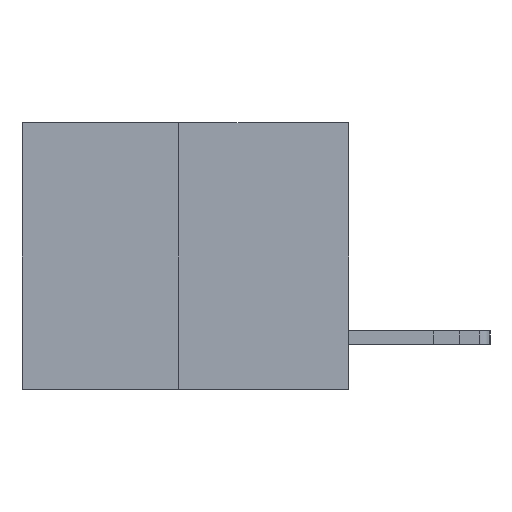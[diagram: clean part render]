
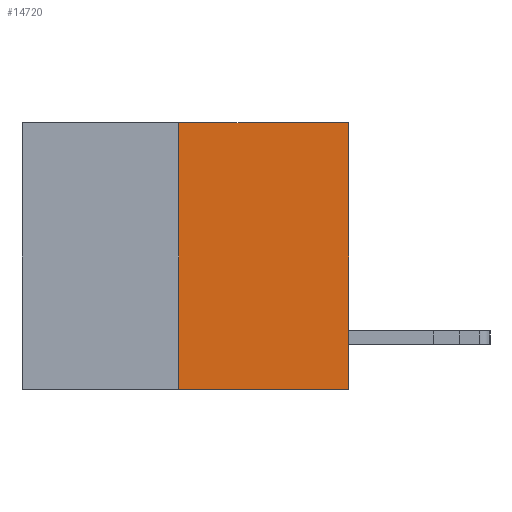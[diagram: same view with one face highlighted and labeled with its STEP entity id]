
A CAD part, left-side view. The second image highlights one B-rep face of the part: STEP entity #14720.
In plain terms, the highlighted planar face has unit normal (-1, 0, 0).
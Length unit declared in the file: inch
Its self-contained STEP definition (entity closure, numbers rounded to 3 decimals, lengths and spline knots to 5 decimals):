
#1725 = EDGE_CURVE ( 'NONE', #3809, #10018, #12631, .T. ) ;
#1791 = CARTESIAN_POINT ( 'NONE',  ( 0., 0.312, 0. ) ) ;
#3809 = VERTEX_POINT ( 'NONE', #7049 ) ;
#4266 = CARTESIAN_POINT ( 'NONE',  ( 0., 0.6, 0. ) ) ;
#4326 = DIRECTION ( 'NONE',  ( 1., 0., 0. ) ) ;
#4959 = ORIENTED_EDGE ( 'NONE', *, *, #5441, .F. ) ;
#5100 = ORIENTED_EDGE ( 'NONE', *, *, #14670, .T. ) ;
#5299 = CARTESIAN_POINT ( 'NONE',  ( 0., 0.6, -0.49 ) ) ;
#5441 = EDGE_CURVE ( 'NONE', #10018, #7235, #14806, .T. ) ;
#5541 = ORIENTED_EDGE ( 'NONE', *, *, #15713, .T. ) ;
#5608 = CARTESIAN_POINT ( 'NONE',  ( 0., 0., -0.49 ) ) ;
#7049 = CARTESIAN_POINT ( 'NONE',  ( 0., 0.312, -0.49 ) ) ;
#7235 = VERTEX_POINT ( 'NONE', #12132 ) ;
#7618 = DIRECTION ( 'NONE',  ( 0., 0., 1. ) ) ;
#7850 = LINE ( 'NONE', #14991, #15889 ) ;
#8002 = CARTESIAN_POINT ( 'NONE',  ( 0., 0.6, 0. ) ) ;
#8866 = VERTEX_POINT ( 'NONE', #5608 ) ;
#9265 = DIRECTION ( 'NONE',  ( 0., 0., -1. ) ) ;
#9460 = LINE ( 'NONE', #5299, #15340 ) ;
#9776 = EDGE_LOOP ( 'NONE', ( #15896, #5100, #5541, #4959 ) ) ;
#10018 = VERTEX_POINT ( 'NONE', #1791 ) ;
#10072 = DIRECTION ( 'NONE',  ( 0., 0., 1. ) ) ;
#10525 = CARTESIAN_POINT ( 'NONE',  ( 0., 0.312, -0.49 ) ) ;
#10681 = VECTOR ( 'NONE', #15390, 39.37008 ) ;
#11904 = PLANE ( 'NONE',  #14398 ) ;
#12132 = CARTESIAN_POINT ( 'NONE',  ( 0., 0., 0. ) ) ;
#12631 = LINE ( 'NONE', #10525, #13017 ) ;
#12973 = FACE_OUTER_BOUND ( 'NONE', #9776, .T. ) ;
#13017 = VECTOR ( 'NONE', #7618, 39.37008 ) ;
#14398 = AXIS2_PLACEMENT_3D ( 'NONE', #8002, #4326, #9265 ) ;
#14670 = EDGE_CURVE ( 'NONE', #3809, #8866, #9460, .T. ) ;
#14720 = ADVANCED_FACE ( 'NONE', ( #12973 ), #11904, .F. ) ;
#14806 = LINE ( 'NONE', #4266, #10681 ) ;
#14991 = CARTESIAN_POINT ( 'NONE',  ( 0., 0., 0. ) ) ;
#15134 = DIRECTION ( 'NONE',  ( 0., -1., 0. ) ) ;
#15340 = VECTOR ( 'NONE', #15134, 39.37008 ) ;
#15390 = DIRECTION ( 'NONE',  ( 0., -1., 0. ) ) ;
#15713 = EDGE_CURVE ( 'NONE', #8866, #7235, #7850, .T. ) ;
#15889 = VECTOR ( 'NONE', #10072, 39.37008 ) ;
#15896 = ORIENTED_EDGE ( 'NONE', *, *, #1725, .F. ) ;
